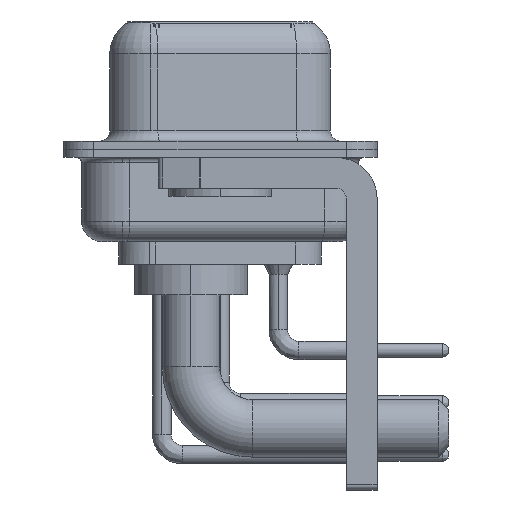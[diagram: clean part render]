
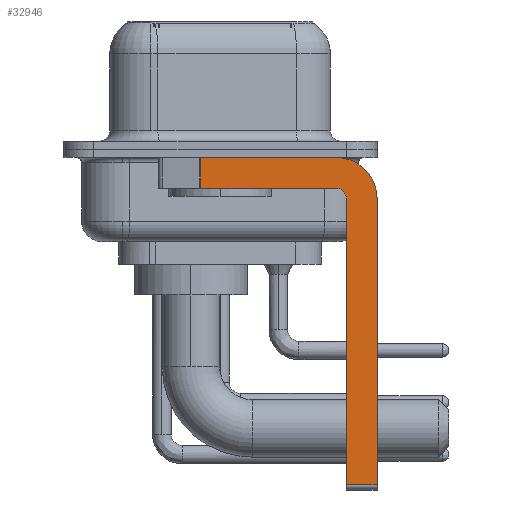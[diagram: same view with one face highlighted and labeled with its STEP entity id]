
A CAD part, left-side view. The second image highlights one B-rep face of the part: STEP entity #32946.
In plain terms, the highlighted planar face has unit normal (-1, 0, 0).
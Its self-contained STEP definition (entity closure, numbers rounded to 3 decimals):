
#676 = CARTESIAN_POINT ( 'NONE',  ( -2.9, -7.65, -16.35 ) ) ;
#946 = EDGE_CURVE ( 'NONE', #19416, #24221, #9082, .T. ) ;
#1444 = CARTESIAN_POINT ( 'NONE',  ( -2.9, -5.65, -1.9 ) ) ;
#1572 = VECTOR ( 'NONE', #9644, 1000. ) ;
#1654 = VERTEX_POINT ( 'NONE', #5477 ) ;
#1718 = LINE ( 'NONE', #14845, #8710 ) ;
#1721 = CARTESIAN_POINT ( 'NONE',  ( -2.9, -5.65, -2.4 ) ) ;
#1814 = AXIS2_PLACEMENT_3D ( 'NONE', #8936, #3890, #8583 ) ;
#3163 = ORIENTED_EDGE ( 'NONE', *, *, #24832, .F. ) ;
#3217 = FACE_OUTER_BOUND ( 'NONE', #27847, .T. ) ;
#3890 = DIRECTION ( 'NONE',  ( 1., 0., 0. ) ) ;
#4194 = CARTESIAN_POINT ( 'NONE',  ( -2.9, -7.65, -2.4 ) ) ;
#5467 = VERTEX_POINT ( 'NONE', #21025 ) ;
#5477 = CARTESIAN_POINT ( 'NONE',  ( -2.9, 0.978, -1.9 ) ) ;
#6638 = VECTOR ( 'NONE', #18564, 1000. ) ;
#7049 = CARTESIAN_POINT ( 'NONE',  ( -2.9, 3., -0.4 ) ) ;
#7100 = DIRECTION ( 'NONE',  ( 0., 0., -1. ) ) ;
#7518 = CARTESIAN_POINT ( 'NONE',  ( -2.9, 0.978, -1.9 ) ) ;
#7590 = VERTEX_POINT ( 'NONE', #4194 ) ;
#8583 = DIRECTION ( 'NONE',  ( 0., 0., -1. ) ) ;
#8710 = VECTOR ( 'NONE', #9790, 1000. ) ;
#8745 = AXIS2_PLACEMENT_3D ( 'NONE', #20634, #30916, #23845 ) ;
#8936 = CARTESIAN_POINT ( 'NONE',  ( -2.9, -5.65, -2.4 ) ) ;
#9082 = LINE ( 'NONE', #7049, #18584 ) ;
#9644 = DIRECTION ( 'NONE',  ( 0., -1., 0. ) ) ;
#9790 = DIRECTION ( 'NONE',  ( 0., 0., 1. ) ) ;
#10394 = ORIENTED_EDGE ( 'NONE', *, *, #29457, .T. ) ;
#10718 = VECTOR ( 'NONE', #20472, 1000. ) ;
#10722 = EDGE_CURVE ( 'NONE', #15833, #5467, #29183, .T. ) ;
#10898 = CARTESIAN_POINT ( 'NONE',  ( -2.9, -5.65, -0.4 ) ) ;
#11800 = ORIENTED_EDGE ( 'NONE', *, *, #22572, .F. ) ;
#12184 = LINE ( 'NONE', #15306, #1572 ) ;
#12414 = LINE ( 'NONE', #7518, #10718 ) ;
#14845 = CARTESIAN_POINT ( 'NONE',  ( -2.9, -6.15, -16.6 ) ) ;
#15306 = CARTESIAN_POINT ( 'NONE',  ( -2.9, -5.65, -16.35 ) ) ;
#15712 = VECTOR ( 'NONE', #24686, 1000. ) ;
#15833 = VERTEX_POINT ( 'NONE', #23851 ) ;
#16534 = CARTESIAN_POINT ( 'NONE',  ( -2.9, -6.15, -16.35 ) ) ;
#16920 = ORIENTED_EDGE ( 'NONE', *, *, #10722, .F. ) ;
#17058 = DIRECTION ( 'NONE',  ( 1., 0., 0. ) ) ;
#18074 = CARTESIAN_POINT ( 'NONE',  ( -2.9, -7.65, -2.4 ) ) ;
#18228 = EDGE_CURVE ( 'NONE', #26575, #27362, #12184, .T. ) ;
#18556 = ORIENTED_EDGE ( 'NONE', *, *, #32094, .F. ) ;
#18564 = DIRECTION ( 'NONE',  ( 0., 0., -1. ) ) ;
#18584 = VECTOR ( 'NONE', #19358, 1000. ) ;
#19289 = LINE ( 'NONE', #1444, #15712 ) ;
#19358 = DIRECTION ( 'NONE',  ( 0., -1., 0. ) ) ;
#19416 = VERTEX_POINT ( 'NONE', #26333 ) ;
#20472 = DIRECTION ( 'NONE',  ( 0., 0., -1. ) ) ;
#20634 = CARTESIAN_POINT ( 'NONE',  ( -2.9, -5.65, -2.4 ) ) ;
#21025 = CARTESIAN_POINT ( 'NONE',  ( -2.9, -5.65, -1.9 ) ) ;
#22209 = EDGE_CURVE ( 'NONE', #7590, #27362, #31353, .T. ) ;
#22310 = CIRCLE ( 'NONE', #28217, 2. ) ;
#22572 = EDGE_CURVE ( 'NONE', #26575, #15833, #1718, .T. ) ;
#23845 = DIRECTION ( 'NONE',  ( 0., 0., 1. ) ) ;
#23851 = CARTESIAN_POINT ( 'NONE',  ( -2.9, -6.15, -2.4 ) ) ;
#24104 = ORIENTED_EDGE ( 'NONE', *, *, #22209, .F. ) ;
#24221 = VERTEX_POINT ( 'NONE', #10898 ) ;
#24686 = DIRECTION ( 'NONE',  ( 0., 1., 0. ) ) ;
#24832 = EDGE_CURVE ( 'NONE', #24221, #7590, #22310, .T. ) ;
#26333 = CARTESIAN_POINT ( 'NONE',  ( -2.9, 0.978, -0.4 ) ) ;
#26575 = VERTEX_POINT ( 'NONE', #16534 ) ;
#26618 = PLANE ( 'NONE',  #1814 ) ;
#27362 = VERTEX_POINT ( 'NONE', #676 ) ;
#27847 = EDGE_LOOP ( 'NONE', ( #29706, #10394, #18556, #16920, #11800, #29196, #24104, #3163 ) ) ;
#28217 = AXIS2_PLACEMENT_3D ( 'NONE', #1721, #17058, #7100 ) ;
#29183 = CIRCLE ( 'NONE', #8745, 0.5 ) ;
#29196 = ORIENTED_EDGE ( 'NONE', *, *, #18228, .T. ) ;
#29457 = EDGE_CURVE ( 'NONE', #19416, #1654, #12414, .T. ) ;
#29706 = ORIENTED_EDGE ( 'NONE', *, *, #946, .F. ) ;
#30916 = DIRECTION ( 'NONE',  ( -1., 0., 0. ) ) ;
#31353 = LINE ( 'NONE', #18074, #6638 ) ;
#32094 = EDGE_CURVE ( 'NONE', #5467, #1654, #19289, .T. ) ;
#32946 = ADVANCED_FACE ( 'NONE', ( #3217 ), #26618, .F. ) ;
